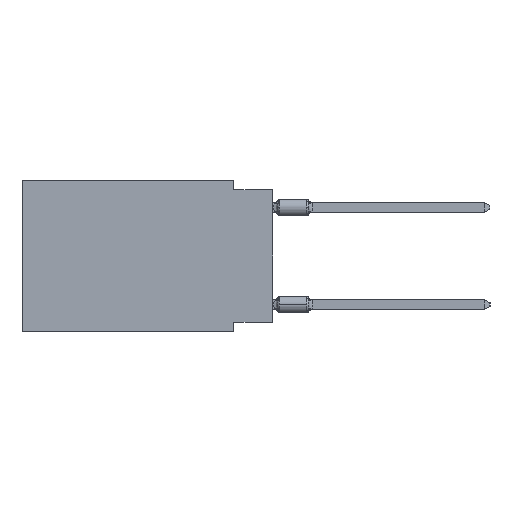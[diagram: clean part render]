
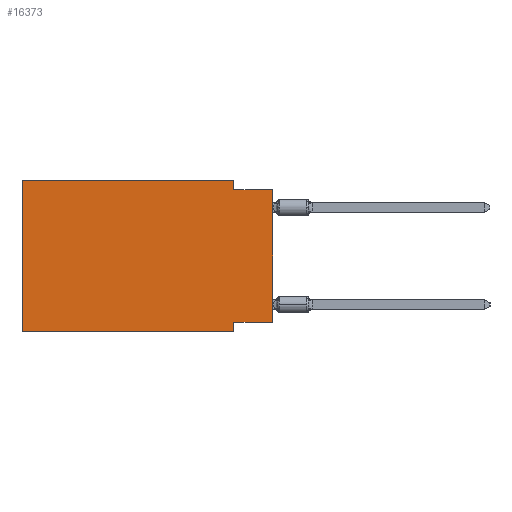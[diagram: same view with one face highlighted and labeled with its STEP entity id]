
A CAD part, left-side view. The second image highlights one B-rep face of the part: STEP entity #16373.
In plain terms, the highlighted planar face has unit normal (-1, 0, 0).
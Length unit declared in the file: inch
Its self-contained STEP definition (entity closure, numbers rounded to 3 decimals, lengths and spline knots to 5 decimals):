
#406 = VECTOR ( 'NONE', #31466, 39.37008 ) ;
#1203 = VERTEX_POINT ( 'NONE', #39202 ) ;
#1846 = CARTESIAN_POINT ( 'NONE',  ( 0., 0.645, 0. ) ) ;
#2119 = DIRECTION ( 'NONE',  ( 0., -1., 0. ) ) ;
#2838 = VECTOR ( 'NONE', #32126, 39.37008 ) ;
#2884 = VECTOR ( 'NONE', #30228, 39.37008 ) ;
#2999 = LINE ( 'NONE', #9422, #17371 ) ;
#3068 = LINE ( 'NONE', #16118, #9561 ) ;
#3466 = CARTESIAN_POINT ( 'NONE',  ( 0., 0., 0. ) ) ;
#3882 = CARTESIAN_POINT ( 'NONE',  ( 0., 0., -0.025 ) ) ;
#3969 = CARTESIAN_POINT ( 'NONE',  ( 0., 0.645, 0. ) ) ;
#4025 = CARTESIAN_POINT ( 'NONE',  ( 0., 0.1, -0.365 ) ) ;
#4120 = LINE ( 'NONE', #35449, #2838 ) ;
#5140 = CARTESIAN_POINT ( 'NONE',  ( 0., 0., -0.365 ) ) ;
#7085 = EDGE_CURVE ( 'NONE', #39509, #24496, #2999, .T. ) ;
#7337 = CARTESIAN_POINT ( 'NONE',  ( 0., 0.1, -0.39 ) ) ;
#7826 = DIRECTION ( 'NONE',  ( 0., -1., 0. ) ) ;
#8267 = LINE ( 'NONE', #5140, #2884 ) ;
#9422 = CARTESIAN_POINT ( 'NONE',  ( 0., 0.645, 0. ) ) ;
#9561 = VECTOR ( 'NONE', #13423, 39.37008 ) ;
#10194 = DIRECTION ( 'NONE',  ( 0., 0., -1. ) ) ;
#12359 = EDGE_CURVE ( 'NONE', #1203, #25364, #3068, .T. ) ;
#12809 = LINE ( 'NONE', #3466, #406 ) ;
#13423 = DIRECTION ( 'NONE',  ( 0., 0., -1. ) ) ;
#13841 = LINE ( 'NONE', #3882, #15702 ) ;
#14108 = ORIENTED_EDGE ( 'NONE', *, *, #12359, .F. ) ;
#14144 = VERTEX_POINT ( 'NONE', #37868 ) ;
#15160 = VERTEX_POINT ( 'NONE', #19504 ) ;
#15702 = VECTOR ( 'NONE', #7826, 39.37008 ) ;
#15747 = EDGE_CURVE ( 'NONE', #15160, #29373, #8267, .T. ) ;
#15792 = CARTESIAN_POINT ( 'NONE',  ( 0., 0.1, -0.025 ) ) ;
#16118 = CARTESIAN_POINT ( 'NONE',  ( 0., 0.1, 0. ) ) ;
#16373 = ADVANCED_FACE ( 'NONE', ( #25934 ), #34878, .F. ) ;
#16421 = DIRECTION ( 'NONE',  ( 1., 0., 0. ) ) ;
#17371 = VECTOR ( 'NONE', #31805, 39.37008 ) ;
#18347 = VERTEX_POINT ( 'NONE', #7337 ) ;
#19504 = CARTESIAN_POINT ( 'NONE',  ( 0., 0., -0.365 ) ) ;
#20896 = ORIENTED_EDGE ( 'NONE', *, *, #39424, .F. ) ;
#21600 = ORIENTED_EDGE ( 'NONE', *, *, #29386, .T. ) ;
#22493 = DIRECTION ( 'NONE',  ( 0., 0., -1. ) ) ;
#23152 = CARTESIAN_POINT ( 'NONE',  ( 0., 0.645, -0.39 ) ) ;
#23332 = EDGE_CURVE ( 'NONE', #29373, #18347, #28116, .T. ) ;
#23943 = VECTOR ( 'NONE', #2119, 39.37008 ) ;
#24496 = VERTEX_POINT ( 'NONE', #1846 ) ;
#24639 = ORIENTED_EDGE ( 'NONE', *, *, #15747, .F. ) ;
#25364 = VERTEX_POINT ( 'NONE', #15792 ) ;
#25934 = FACE_OUTER_BOUND ( 'NONE', #30432, .T. ) ;
#26968 = ORIENTED_EDGE ( 'NONE', *, *, #40538, .T. ) ;
#27080 = ORIENTED_EDGE ( 'NONE', *, *, #23332, .F. ) ;
#28116 = LINE ( 'NONE', #38269, #40240 ) ;
#29373 = VERTEX_POINT ( 'NONE', #4025 ) ;
#29386 = EDGE_CURVE ( 'NONE', #39509, #18347, #33859, .T. ) ;
#30186 = EDGE_CURVE ( 'NONE', #24496, #1203, #4120, .T. ) ;
#30228 = DIRECTION ( 'NONE',  ( 0., 1., 0. ) ) ;
#30432 = EDGE_LOOP ( 'NONE', ( #26968, #20896, #14108, #36374, #33230, #21600, #27080, #24639 ) ) ;
#31390 = AXIS2_PLACEMENT_3D ( 'NONE', #3969, #16421, #10194 ) ;
#31466 = DIRECTION ( 'NONE',  ( 0., 0., 1. ) ) ;
#31805 = DIRECTION ( 'NONE',  ( 0., 0., 1. ) ) ;
#32126 = DIRECTION ( 'NONE',  ( 0., -1., 0. ) ) ;
#33230 = ORIENTED_EDGE ( 'NONE', *, *, #7085, .F. ) ;
#33859 = LINE ( 'NONE', #40483, #23943 ) ;
#34878 = PLANE ( 'NONE',  #31390 ) ;
#35449 = CARTESIAN_POINT ( 'NONE',  ( 0., 0.645, 0. ) ) ;
#36374 = ORIENTED_EDGE ( 'NONE', *, *, #30186, .F. ) ;
#37868 = CARTESIAN_POINT ( 'NONE',  ( 0., 0., -0.025 ) ) ;
#38269 = CARTESIAN_POINT ( 'NONE',  ( 0., 0.1, -0.39 ) ) ;
#39202 = CARTESIAN_POINT ( 'NONE',  ( 0., 0.1, 0. ) ) ;
#39424 = EDGE_CURVE ( 'NONE', #25364, #14144, #13841, .T. ) ;
#39509 = VERTEX_POINT ( 'NONE', #23152 ) ;
#40240 = VECTOR ( 'NONE', #22493, 39.37008 ) ;
#40483 = CARTESIAN_POINT ( 'NONE',  ( 0., 0.645, -0.39 ) ) ;
#40538 = EDGE_CURVE ( 'NONE', #15160, #14144, #12809, .T. ) ;
